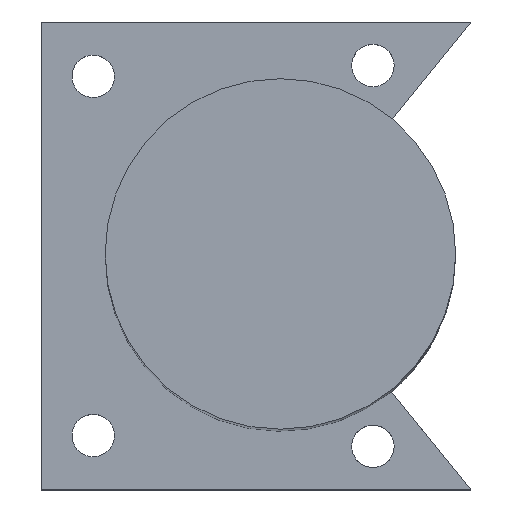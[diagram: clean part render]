
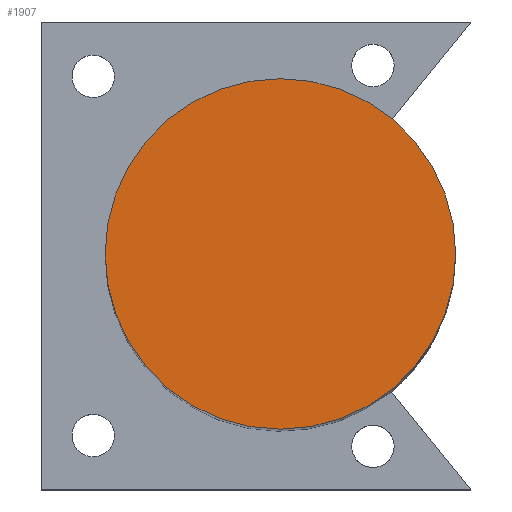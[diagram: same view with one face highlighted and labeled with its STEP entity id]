
A CAD part, top view. The second image highlights one B-rep face of the part: STEP entity #1907.
In plain terms, the highlighted planar face has unit normal (0, 0, 1).
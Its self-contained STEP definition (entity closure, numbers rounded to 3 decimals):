
#623 = CYLINDRICAL_SURFACE('',#624,16.108);
#624 = AXIS2_PLACEMENT_3D('',#625,#626,#627);
#625 = CARTESIAN_POINT('',(-17.5,-21.5,0.));
#626 = DIRECTION('',(0.,0.,-1.));
#627 = DIRECTION('',(1.,0.,0.));
#1356 = VERTEX_POINT('',#1357);
#1357 = CARTESIAN_POINT('',(-1.392,-21.5,111.));
#1378 = EDGE_CURVE('',#1356,#1356,#1379,.T.);
#1379 = SURFACE_CURVE('',#1380,(#1385,#1392),.PCURVE_S1.);
#1380 = CIRCLE('',#1381,16.108);
#1381 = AXIS2_PLACEMENT_3D('',#1382,#1383,#1384);
#1382 = CARTESIAN_POINT('',(-17.5,-21.5,111.));
#1383 = DIRECTION('',(0.,0.,1.));
#1384 = DIRECTION('',(1.,0.,0.));
#1385 = PCURVE('',#623,#1386);
#1386 = DEFINITIONAL_REPRESENTATION('',(#1387),#1391);
#1387 = LINE('',#1388,#1389);
#1388 = CARTESIAN_POINT('',(0.,-111.));
#1389 = VECTOR('',#1390,1.);
#1390 = DIRECTION('',(-1.,0.));
#1391 = ( GEOMETRIC_REPRESENTATION_CONTEXT(2) 
PARAMETRIC_REPRESENTATION_CONTEXT() REPRESENTATION_CONTEXT('2D SPACE',''
  ) );
#1392 = PCURVE('',#1393,#1398);
#1393 = PLANE('',#1394);
#1394 = AXIS2_PLACEMENT_3D('',#1395,#1396,#1397);
#1395 = CARTESIAN_POINT('',(-1.392,-21.5,111.));
#1396 = DIRECTION('',(0.,0.,-1.));
#1397 = DIRECTION('',(-1.,0.,0.));
#1398 = DEFINITIONAL_REPRESENTATION('',(#1399),#1407);
#1399 = ( BOUNDED_CURVE() B_SPLINE_CURVE(2,(#1400,#1401,#1402,#1403,
#1404,#1405,#1406),.UNSPECIFIED.,.F.,.F.) B_SPLINE_CURVE_WITH_KNOTS((1,2
    ,2,2,2,1),(-2.094,0.,2.094,4.189,
6.283,8.378),.UNSPECIFIED.) CURVE() 
GEOMETRIC_REPRESENTATION_ITEM() RATIONAL_B_SPLINE_CURVE((1.,0.5,1.,0.5,
1.,0.5,1.)) REPRESENTATION_ITEM('') );
#1400 = CARTESIAN_POINT('',(0.,0.));
#1401 = CARTESIAN_POINT('',(0.,27.9));
#1402 = CARTESIAN_POINT('',(24.162,13.95));
#1403 = CARTESIAN_POINT('',(48.324,0.));
#1404 = CARTESIAN_POINT('',(24.162,-13.95));
#1405 = CARTESIAN_POINT('',(0.,-27.9));
#1406 = CARTESIAN_POINT('',(0.,0.));
#1407 = ( GEOMETRIC_REPRESENTATION_CONTEXT(2) 
PARAMETRIC_REPRESENTATION_CONTEXT() REPRESENTATION_CONTEXT('2D SPACE',''
  ) );
#1907 = ADVANCED_FACE('',(#1908),#1393,.F.);
#1908 = FACE_BOUND('',#1909,.T.);
#1909 = EDGE_LOOP('',(#1910));
#1910 = ORIENTED_EDGE('',*,*,#1378,.T.);
